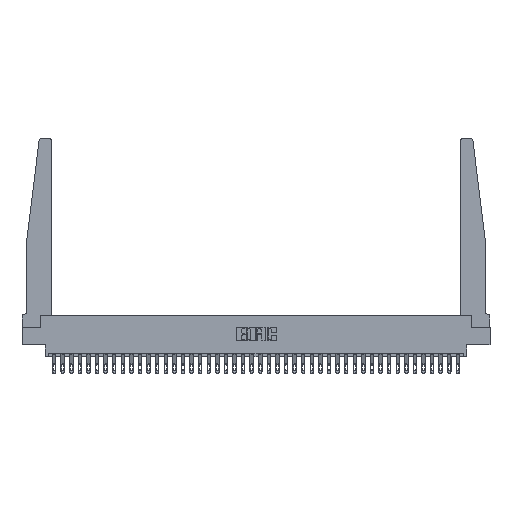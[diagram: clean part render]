
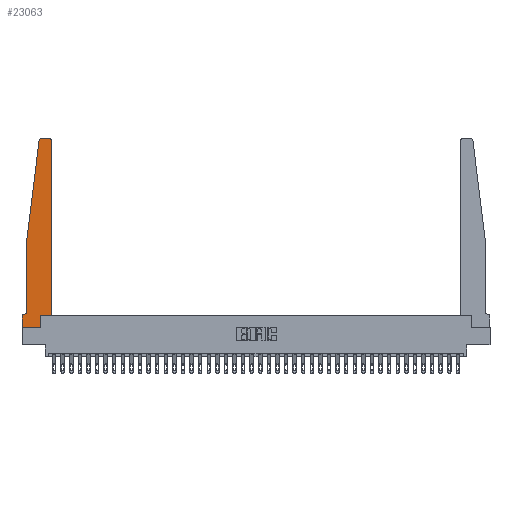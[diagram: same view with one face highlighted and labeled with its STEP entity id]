
A CAD part, top view. The second image highlights one B-rep face of the part: STEP entity #23063.
In plain terms, the highlighted planar face has unit normal (0, 0, 1).
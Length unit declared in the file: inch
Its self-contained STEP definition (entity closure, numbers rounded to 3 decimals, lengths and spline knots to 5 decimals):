
#484 = CARTESIAN_POINT ( 'NONE',  ( 0.065, 1.25, 0.37 ) ) ;
#717 = CARTESIAN_POINT ( 'NONE',  ( 0.27653, 2.75, 0.37 ) ) ;
#898 = DIRECTION ( 'NONE',  ( 0., 0., 1. ) ) ;
#957 = CARTESIAN_POINT ( 'NONE',  ( 0., 0., 0.37 ) ) ;
#1811 = CARTESIAN_POINT ( 'NONE',  ( 0.065, 0.2375, 0.37 ) ) ;
#2941 = ORIENTED_EDGE ( 'NONE', *, *, #9887, .T. ) ;
#3005 = VERTEX_POINT ( 'NONE', #28026 ) ;
#3160 = AXIS2_PLACEMENT_3D ( 'NONE', #24029, #4233, #23479 ) ;
#3852 = DIRECTION ( 'NONE',  ( 1., 0., 0. ) ) ;
#4136 = DIRECTION ( 'NONE',  ( 0., 1., 0. ) ) ;
#4233 = DIRECTION ( 'NONE',  ( 0., 0., 1. ) ) ;
#4547 = EDGE_CURVE ( 'NONE', #11847, #24429, #15620, .T. ) ;
#4815 = EDGE_CURVE ( 'NONE', #3005, #21513, #29012, .T. ) ;
#4908 = ORIENTED_EDGE ( 'NONE', *, *, #31395, .T. ) ;
#5589 = VERTEX_POINT ( 'NONE', #19970 ) ;
#5779 = DIRECTION ( 'NONE',  ( 0., 1., 0. ) ) ;
#6876 = LINE ( 'NONE', #29212, #24604 ) ;
#7280 = AXIS2_PLACEMENT_3D ( 'NONE', #9716, #898, #3852 ) ;
#7606 = DIRECTION ( 'NONE',  ( -1., 0., 0. ) ) ;
#7670 = LINE ( 'NONE', #27096, #26356 ) ;
#7684 = CARTESIAN_POINT ( 'NONE',  ( 0.2605, 0., 0.37 ) ) ;
#7813 = EDGE_CURVE ( 'NONE', #14914, #24709, #6876, .T. ) ;
#7866 = DIRECTION ( 'NONE',  ( 0., 0., 1. ) ) ;
#8561 = LINE ( 'NONE', #484, #35694 ) ;
#8721 = EDGE_CURVE ( 'NONE', #26601, #5589, #30503, .T. ) ;
#8968 = EDGE_LOOP ( 'NONE', ( #14859, #27871, #13916, #27520, #34189, #32976, #34087, #18890, #18806, #4908, #20989, #2941 ) ) ;
#9074 = DIRECTION ( 'NONE',  ( 1., 0., 0. ) ) ;
#9224 = VERTEX_POINT ( 'NONE', #957 ) ;
#9622 = CIRCLE ( 'NONE', #7280, 0.03 ) ;
#9716 = CARTESIAN_POINT ( 'NONE',  ( 0.27653, 2.72, 0.37 ) ) ;
#9718 = LINE ( 'NONE', #23465, #35097 ) ;
#9887 = EDGE_CURVE ( 'NONE', #5589, #3005, #33603, .T. ) ;
#11290 = CARTESIAN_POINT ( 'NONE',  ( 0.425, 0.18, 0.37 ) ) ;
#11709 = EDGE_CURVE ( 'NONE', #21513, #35078, #9622, .T. ) ;
#11847 = VERTEX_POINT ( 'NONE', #1811 ) ;
#11936 = VERTEX_POINT ( 'NONE', #22692 ) ;
#12444 = VECTOR ( 'NONE', #29999, 39.37008 ) ;
#12490 = EDGE_CURVE ( 'NONE', #9224, #14914, #17508, .T. ) ;
#12699 = AXIS2_PLACEMENT_3D ( 'NONE', #18981, #32694, #7606 ) ;
#13186 = DIRECTION ( 'NONE',  ( -1., 0., 0. ) ) ;
#13205 = VECTOR ( 'NONE', #9074, 39.37008 ) ;
#13916 = ORIENTED_EDGE ( 'NONE', *, *, #20538, .T. ) ;
#14614 = CARTESIAN_POINT ( 'NONE',  ( 0.015, 0.1875, 0.37 ) ) ;
#14859 = ORIENTED_EDGE ( 'NONE', *, *, #4815, .T. ) ;
#14914 = VERTEX_POINT ( 'NONE', #7684 ) ;
#15620 = CIRCLE ( 'NONE', #12699, 0.05 ) ;
#15931 = AXIS2_PLACEMENT_3D ( 'NONE', #18883, #7866, #16300 ) ;
#16137 = VERTEX_POINT ( 'NONE', #34485 ) ;
#16275 = LINE ( 'NONE', #25569, #12444 ) ;
#16300 = DIRECTION ( 'NONE',  ( 1., 0., 0. ) ) ;
#17508 = LINE ( 'NONE', #23011, #13205 ) ;
#17788 = DIRECTION ( 'NONE',  ( 0., -1., 0. ) ) ;
#18082 = LINE ( 'NONE', #23391, #29296 ) ;
#18806 = ORIENTED_EDGE ( 'NONE', *, *, #7813, .T. ) ;
#18883 = CARTESIAN_POINT ( 'NONE',  ( 0., 0.1875, 0.37 ) ) ;
#18890 = ORIENTED_EDGE ( 'NONE', *, *, #12490, .T. ) ;
#18981 = CARTESIAN_POINT ( 'NONE',  ( 0.015, 0.2375, 0.37 ) ) ;
#19526 = CARTESIAN_POINT ( 'NONE',  ( 0.24675, 2.72367, 0.37 ) ) ;
#19579 = DIRECTION ( 'NONE',  ( -0.122, -0.992, 0. ) ) ;
#19970 = CARTESIAN_POINT ( 'NONE',  ( 0.425, 2.72, 0.37 ) ) ;
#20200 = EDGE_CURVE ( 'NONE', #11936, #9224, #9718, .T. ) ;
#20329 = EDGE_CURVE ( 'NONE', #24429, #11936, #7670, .T. ) ;
#20538 = EDGE_CURVE ( 'NONE', #35078, #16137, #8561, .T. ) ;
#20989 = ORIENTED_EDGE ( 'NONE', *, *, #8721, .T. ) ;
#21334 = CARTESIAN_POINT ( 'NONE',  ( 0.25, 2.75, 0.37 ) ) ;
#21513 = VERTEX_POINT ( 'NONE', #717 ) ;
#22692 = CARTESIAN_POINT ( 'NONE',  ( 0., 0.1875, 0.37 ) ) ;
#23011 = CARTESIAN_POINT ( 'NONE',  ( 0., 0., 0.37 ) ) ;
#23063 = ADVANCED_FACE ( 'NONE', ( #32953 ), #27819, .T. ) ;
#23391 = CARTESIAN_POINT ( 'NONE',  ( 0.065, 1.25, 0.37 ) ) ;
#23465 = CARTESIAN_POINT ( 'NONE',  ( 0., 0., 0.37 ) ) ;
#23479 = DIRECTION ( 'NONE',  ( 1., 0., 0. ) ) ;
#23570 = DIRECTION ( 'NONE',  ( 0., -1., 0. ) ) ;
#23948 = VECTOR ( 'NONE', #5779, 39.37008 ) ;
#24029 = CARTESIAN_POINT ( 'NONE',  ( 0.395, 2.72, 0.37 ) ) ;
#24429 = VERTEX_POINT ( 'NONE', #14614 ) ;
#24604 = VECTOR ( 'NONE', #4136, 39.37008 ) ;
#24709 = VERTEX_POINT ( 'NONE', #25882 ) ;
#25569 = CARTESIAN_POINT ( 'NONE',  ( 0.425, 0.18, 0.37 ) ) ;
#25882 = CARTESIAN_POINT ( 'NONE',  ( 0.2605, 0.18, 0.37 ) ) ;
#26159 = VECTOR ( 'NONE', #26282, 39.37008 ) ;
#26282 = DIRECTION ( 'NONE',  ( -1., 0., 0. ) ) ;
#26356 = VECTOR ( 'NONE', #13186, 39.37008 ) ;
#26601 = VERTEX_POINT ( 'NONE', #30550 ) ;
#27096 = CARTESIAN_POINT ( 'NONE',  ( 0.065, 0.1875, 0.37 ) ) ;
#27438 = EDGE_CURVE ( 'NONE', #16137, #11847, #18082, .T. ) ;
#27520 = ORIENTED_EDGE ( 'NONE', *, *, #27438, .T. ) ;
#27819 = PLANE ( 'NONE',  #15931 ) ;
#27871 = ORIENTED_EDGE ( 'NONE', *, *, #11709, .T. ) ;
#28026 = CARTESIAN_POINT ( 'NONE',  ( 0.395, 2.75, 0.37 ) ) ;
#29012 = LINE ( 'NONE', #21334, #26159 ) ;
#29212 = CARTESIAN_POINT ( 'NONE',  ( 0.2605, 0.18, 0.37 ) ) ;
#29296 = VECTOR ( 'NONE', #23570, 39.37008 ) ;
#29999 = DIRECTION ( 'NONE',  ( 1., 0., 0. ) ) ;
#30503 = LINE ( 'NONE', #11290, #23948 ) ;
#30550 = CARTESIAN_POINT ( 'NONE',  ( 0.425, 0.18, 0.37 ) ) ;
#31395 = EDGE_CURVE ( 'NONE', #24709, #26601, #16275, .T. ) ;
#32694 = DIRECTION ( 'NONE',  ( 0., 0., -1. ) ) ;
#32953 = FACE_OUTER_BOUND ( 'NONE', #8968, .T. ) ;
#32976 = ORIENTED_EDGE ( 'NONE', *, *, #20329, .T. ) ;
#33603 = CIRCLE ( 'NONE', #3160, 0.03 ) ;
#34087 = ORIENTED_EDGE ( 'NONE', *, *, #20200, .T. ) ;
#34189 = ORIENTED_EDGE ( 'NONE', *, *, #4547, .T. ) ;
#34485 = CARTESIAN_POINT ( 'NONE',  ( 0.065, 1.25, 0.37 ) ) ;
#35078 = VERTEX_POINT ( 'NONE', #19526 ) ;
#35097 = VECTOR ( 'NONE', #17788, 39.37008 ) ;
#35694 = VECTOR ( 'NONE', #19579, 39.37008 ) ;
